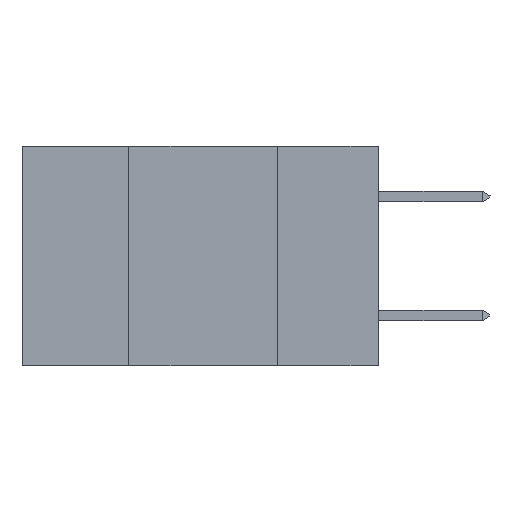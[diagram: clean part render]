
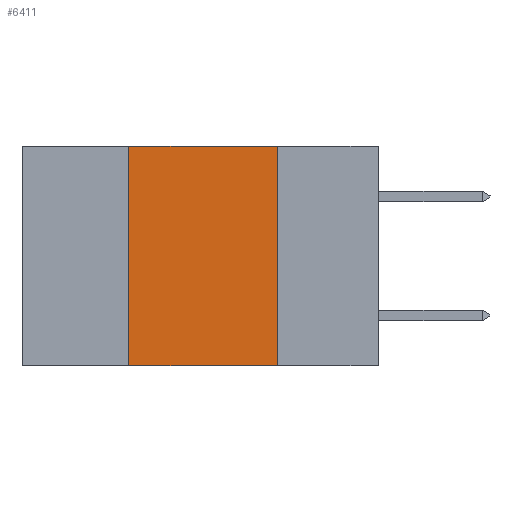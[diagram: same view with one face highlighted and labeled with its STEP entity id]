
A CAD part, left-side view. The second image highlights one B-rep face of the part: STEP entity #6411.
In plain terms, the highlighted planar face has unit normal (-1, 0, 0).
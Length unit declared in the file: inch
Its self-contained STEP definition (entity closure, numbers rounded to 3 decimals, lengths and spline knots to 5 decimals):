
#1632 = DIRECTION ( 'NONE',  ( 0., 0., -1. ) ) ;
#2304 = VERTEX_POINT ( 'NONE', #4438 ) ;
#2338 = VERTEX_POINT ( 'NONE', #5718 ) ;
#3091 = VECTOR ( 'NONE', #5656, 39.37008 ) ;
#3124 = EDGE_LOOP ( 'NONE', ( #13525, #4410, #19858, #6785 ) ) ;
#4410 = ORIENTED_EDGE ( 'NONE', *, *, #14259, .F. ) ;
#4438 = CARTESIAN_POINT ( 'NONE',  ( 0., 0.42, 0. ) ) ;
#4669 = LINE ( 'NONE', #14252, #13153 ) ;
#5656 = DIRECTION ( 'NONE',  ( 0., -1., 0. ) ) ;
#5718 = CARTESIAN_POINT ( 'NONE',  ( 0., 0.17, -0.37 ) ) ;
#6411 = ADVANCED_FACE ( 'NONE', ( #9373 ), #14478, .F. ) ;
#6785 = ORIENTED_EDGE ( 'NONE', *, *, #19168, .T. ) ;
#6845 = EDGE_CURVE ( 'NONE', #18519, #2338, #4669, .T. ) ;
#7853 = VECTOR ( 'NONE', #14811, 39.37008 ) ;
#8225 = EDGE_CURVE ( 'NONE', #10718, #2304, #10062, .T. ) ;
#8417 = CARTESIAN_POINT ( 'NONE',  ( 0., 0.6, -0.37 ) ) ;
#9373 = FACE_OUTER_BOUND ( 'NONE', #3124, .T. ) ;
#9471 = CARTESIAN_POINT ( 'NONE',  ( 0., 0.6, 0. ) ) ;
#10062 = LINE ( 'NONE', #11643, #18886 ) ;
#10169 = AXIS2_PLACEMENT_3D ( 'NONE', #9471, #12514, #17320 ) ;
#10441 = CARTESIAN_POINT ( 'NONE',  ( 0., 0.6, 0. ) ) ;
#10718 = VERTEX_POINT ( 'NONE', #15971 ) ;
#11643 = CARTESIAN_POINT ( 'NONE',  ( 0., 0.42, -0.37 ) ) ;
#12108 = LINE ( 'NONE', #10441, #3091 ) ;
#12514 = DIRECTION ( 'NONE',  ( 1., 0., 0. ) ) ;
#13153 = VECTOR ( 'NONE', #1632, 39.37008 ) ;
#13525 = ORIENTED_EDGE ( 'NONE', *, *, #6845, .F. ) ;
#14252 = CARTESIAN_POINT ( 'NONE',  ( 0., 0.17, -0.37 ) ) ;
#14259 = EDGE_CURVE ( 'NONE', #2304, #18519, #12108, .T. ) ;
#14311 = CARTESIAN_POINT ( 'NONE',  ( 0., 0.17, 0. ) ) ;
#14478 = PLANE ( 'NONE',  #10169 ) ;
#14811 = DIRECTION ( 'NONE',  ( 0., -1., 0. ) ) ;
#15971 = CARTESIAN_POINT ( 'NONE',  ( 0., 0.42, -0.37 ) ) ;
#16342 = DIRECTION ( 'NONE',  ( 0., 0., 1. ) ) ;
#16382 = LINE ( 'NONE', #8417, #7853 ) ;
#17320 = DIRECTION ( 'NONE',  ( 0., 0., -1. ) ) ;
#18519 = VERTEX_POINT ( 'NONE', #14311 ) ;
#18886 = VECTOR ( 'NONE', #16342, 39.37008 ) ;
#19168 = EDGE_CURVE ( 'NONE', #10718, #2338, #16382, .T. ) ;
#19858 = ORIENTED_EDGE ( 'NONE', *, *, #8225, .F. ) ;
